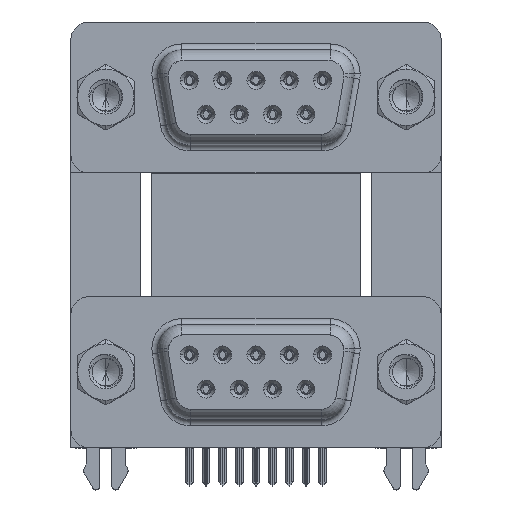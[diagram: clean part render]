
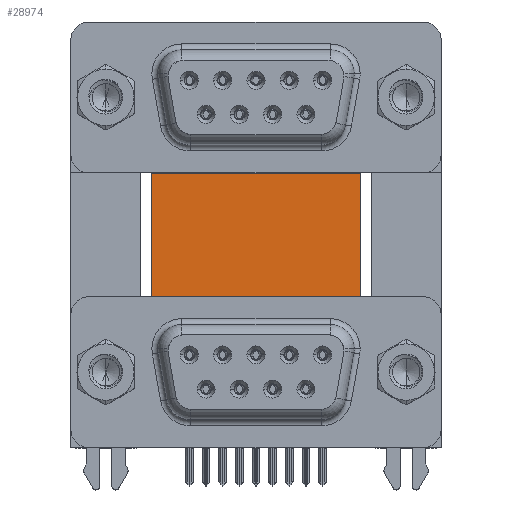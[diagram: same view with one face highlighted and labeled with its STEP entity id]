
A CAD part, top view. The second image highlights one B-rep face of the part: STEP entity #28974.
In plain terms, the highlighted planar face has unit normal (0, 0, 1).
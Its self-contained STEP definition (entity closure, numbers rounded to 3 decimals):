
#599 = EDGE_CURVE ( 'NONE', #46552, #9053, #5927, .T. ) ;
#2827 = AXIS2_PLACEMENT_3D ( 'NONE', #7477, #14728, #30016 ) ;
#3379 = CARTESIAN_POINT ( 'NONE',  ( 22.09, -3.735, -12. ) ) ;
#3689 = VECTOR ( 'NONE', #22163, 1000. ) ;
#4373 = CARTESIAN_POINT ( 'NONE',  ( 22.59, -4.635, -12. ) ) ;
#5513 = EDGE_CURVE ( 'NONE', #45358, #39852, #47301, .T. ) ;
#5675 = DIRECTION ( 'NONE',  ( 1., 0., 0. ) ) ;
#5927 = LINE ( 'NONE', #9438, #7974 ) ;
#7058 = CARTESIAN_POINT ( 'NONE',  ( 22.09, -4.635, -12. ) ) ;
#7274 = CARTESIAN_POINT ( 'NONE',  ( 2.9, -4.635, -12. ) ) ;
#7477 = CARTESIAN_POINT ( 'NONE',  ( 3.79, 16.585, -12. ) ) ;
#7974 = VECTOR ( 'NONE', #5675, 1000. ) ;
#9053 = VERTEX_POINT ( 'NONE', #9334 ) ;
#9334 = CARTESIAN_POINT ( 'NONE',  ( 22.09, -3.735, -12. ) ) ;
#9438 = CARTESIAN_POINT ( 'NONE',  ( 3.79, -3.735, -12. ) ) ;
#9475 = CARTESIAN_POINT ( 'NONE',  ( 3.79, 16.585, -12. ) ) ;
#9960 = CARTESIAN_POINT ( 'NONE',  ( 22.09, -4.635, -12. ) ) ;
#11237 = FACE_OUTER_BOUND ( 'NONE', #34355, .T. ) ;
#11801 = VERTEX_POINT ( 'NONE', #9960 ) ;
#12993 = CARTESIAN_POINT ( 'NONE',  ( 21.2, 16.585, -12. ) ) ;
#14151 = DIRECTION ( 'NONE',  ( 0., 1., 0. ) ) ;
#14728 = DIRECTION ( 'NONE',  ( 0., 0., -1. ) ) ;
#16092 = VECTOR ( 'NONE', #30189, 1000. ) ;
#16974 = ORIENTED_EDGE ( 'NONE', *, *, #5513, .F. ) ;
#17566 = ORIENTED_EDGE ( 'NONE', *, *, #30653, .T. ) ;
#17728 = LINE ( 'NONE', #9475, #37398 ) ;
#17923 = LINE ( 'NONE', #33197, #35341 ) ;
#18670 = DIRECTION ( 'NONE',  ( -0.336, 0.942, 0. ) ) ;
#18681 = CARTESIAN_POINT ( 'NONE',  ( 21.2, -0.735, -12. ) ) ;
#19870 = VERTEX_POINT ( 'NONE', #49518 ) ;
#20915 = EDGE_CURVE ( 'NONE', #39024, #39852, #45725, .T. ) ;
#21367 = LINE ( 'NONE', #7058, #38976 ) ;
#21409 = VECTOR ( 'NONE', #31474, 1000. ) ;
#21412 = EDGE_CURVE ( 'NONE', #19870, #25626, #33888, .T. ) ;
#21711 = LINE ( 'NONE', #48484, #16092 ) ;
#21899 = ORIENTED_EDGE ( 'NONE', *, *, #45798, .T. ) ;
#22163 = DIRECTION ( 'NONE',  ( 0., -1., 0. ) ) ;
#22870 = CARTESIAN_POINT ( 'NONE',  ( 22.59, -4.635, -12. ) ) ;
#24333 = VERTEX_POINT ( 'NONE', #29042 ) ;
#25048 = ORIENTED_EDGE ( 'NONE', *, *, #32725, .T. ) ;
#25626 = VERTEX_POINT ( 'NONE', #7274 ) ;
#26306 = VERTEX_POINT ( 'NONE', #46537 ) ;
#26430 = VECTOR ( 'NONE', #18670, 1000. ) ;
#26647 = DIRECTION ( 'NONE',  ( 1., 0., 0. ) ) ;
#28036 = VECTOR ( 'NONE', #26647, 1000. ) ;
#28285 = DIRECTION ( 'NONE',  ( 0., -1., 0. ) ) ;
#28974 = ADVANCED_FACE ( 'NONE', ( #11237 ), #45552, .F. ) ;
#29042 = CARTESIAN_POINT ( 'NONE',  ( 3.79, -0.735, -12. ) ) ;
#29129 = ORIENTED_EDGE ( 'NONE', *, *, #39870, .F. ) ;
#30016 = DIRECTION ( 'NONE',  ( -1., 0., 0. ) ) ;
#30189 = DIRECTION ( 'NONE',  ( 1., 0., 0. ) ) ;
#30653 = EDGE_CURVE ( 'NONE', #9053, #11801, #37692, .T. ) ;
#30975 = LINE ( 'NONE', #38255, #21409 ) ;
#31474 = DIRECTION ( 'NONE',  ( -0.336, -0.942, 0. ) ) ;
#32725 = EDGE_CURVE ( 'NONE', #24333, #19870, #30975, .T. ) ;
#33011 = DIRECTION ( 'NONE',  ( 0., -1., 0. ) ) ;
#33197 = CARTESIAN_POINT ( 'NONE',  ( 2.9, -3.735, -12. ) ) ;
#33888 = LINE ( 'NONE', #49147, #28036 ) ;
#34355 = EDGE_LOOP ( 'NONE', ( #40083, #17566, #21899, #48614, #16974, #29129, #43439, #25048, #49343, #34537 ) ) ;
#34537 = ORIENTED_EDGE ( 'NONE', *, *, #43106, .T. ) ;
#35341 = VECTOR ( 'NONE', #14151, 1000. ) ;
#37398 = VECTOR ( 'NONE', #33011, 1000. ) ;
#37692 = LINE ( 'NONE', #3379, #3689 ) ;
#38255 = CARTESIAN_POINT ( 'NONE',  ( 2.4, -4.635, -12. ) ) ;
#38976 = VECTOR ( 'NONE', #48882, 1000. ) ;
#39024 = VERTEX_POINT ( 'NONE', #22870 ) ;
#39852 = VERTEX_POINT ( 'NONE', #18681 ) ;
#39870 = EDGE_CURVE ( 'NONE', #26306, #45358, #21711, .T. ) ;
#40083 = ORIENTED_EDGE ( 'NONE', *, *, #599, .T. ) ;
#43106 = EDGE_CURVE ( 'NONE', #25626, #46552, #17923, .T. ) ;
#43439 = ORIENTED_EDGE ( 'NONE', *, *, #46542, .T. ) ;
#44770 = CARTESIAN_POINT ( 'NONE',  ( 2.9, -3.735, -12. ) ) ;
#45358 = VERTEX_POINT ( 'NONE', #49177 ) ;
#45552 = PLANE ( 'NONE',  #2827 ) ;
#45725 = LINE ( 'NONE', #4373, #26430 ) ;
#45798 = EDGE_CURVE ( 'NONE', #11801, #39024, #21367, .T. ) ;
#46537 = CARTESIAN_POINT ( 'NONE',  ( 3.79, 16.585, -12. ) ) ;
#46542 = EDGE_CURVE ( 'NONE', #26306, #24333, #17728, .T. ) ;
#46552 = VERTEX_POINT ( 'NONE', #44770 ) ;
#47301 = LINE ( 'NONE', #12993, #47881 ) ;
#47881 = VECTOR ( 'NONE', #28285, 1000. ) ;
#48484 = CARTESIAN_POINT ( 'NONE',  ( 3.79, 16.585, -12. ) ) ;
#48614 = ORIENTED_EDGE ( 'NONE', *, *, #20915, .T. ) ;
#48882 = DIRECTION ( 'NONE',  ( 1., 0., 0. ) ) ;
#49147 = CARTESIAN_POINT ( 'NONE',  ( 2.9, -4.635, -12. ) ) ;
#49177 = CARTESIAN_POINT ( 'NONE',  ( 21.2, 16.585, -12. ) ) ;
#49343 = ORIENTED_EDGE ( 'NONE', *, *, #21412, .T. ) ;
#49518 = CARTESIAN_POINT ( 'NONE',  ( 2.4, -4.635, -12. ) ) ;
